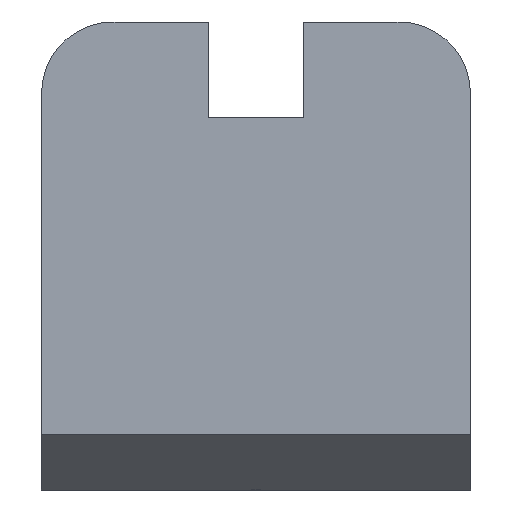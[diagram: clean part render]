
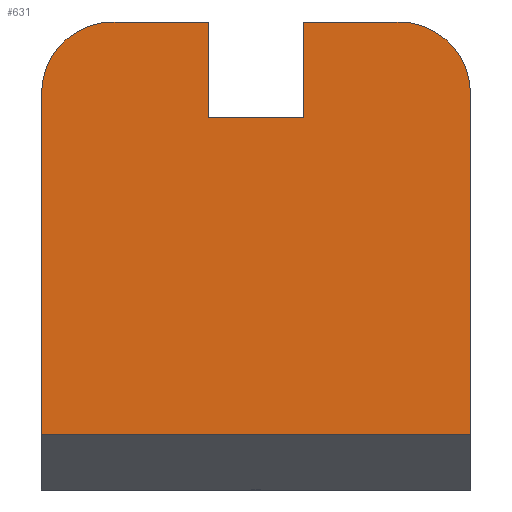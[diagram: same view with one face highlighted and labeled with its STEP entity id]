
A CAD part, top view. The second image highlights one B-rep face of the part: STEP entity #631.
In plain terms, the highlighted planar face has unit normal (0, 0, 1).
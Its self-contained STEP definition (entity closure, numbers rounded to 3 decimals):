
#15 = CARTESIAN_POINT ( 'NONE',  ( 21.823, 44.547, 4. ) ) ;
#56 = VERTEX_POINT ( 'NONE', #776 ) ;
#60 = LINE ( 'NONE', #400, #99 ) ;
#68 = EDGE_CURVE ( 'NONE', #308, #432, #564, .T. ) ;
#85 = EDGE_CURVE ( 'NONE', #425, #56, #176, .T. ) ;
#99 = VECTOR ( 'NONE', #409, 1000. ) ;
#122 = ORIENTED_EDGE ( 'NONE', *, *, #85, .T. ) ;
#123 = CIRCLE ( 'NONE', #684, 3. ) ;
#139 = ORIENTED_EDGE ( 'NONE', *, *, #194, .F. ) ;
#146 = EDGE_CURVE ( 'NONE', #341, #425, #325, .T. ) ;
#150 = VECTOR ( 'NONE', #211, 1000. ) ;
#164 = ORIENTED_EDGE ( 'NONE', *, *, #462, .T. ) ;
#174 = EDGE_CURVE ( 'NONE', #188, #56, #60, .T. ) ;
#176 = LINE ( 'NONE', #394, #235 ) ;
#185 = EDGE_CURVE ( 'NONE', #264, #188, #372, .T. ) ;
#186 = VERTEX_POINT ( 'NONE', #480 ) ;
#188 = VERTEX_POINT ( 'NONE', #617 ) ;
#194 = EDGE_CURVE ( 'NONE', #308, #264, #758, .T. ) ;
#195 = VERTEX_POINT ( 'NONE', #217 ) ;
#210 = DIRECTION ( 'NONE',  ( 1., 0., 0. ) ) ;
#211 = DIRECTION ( 'NONE',  ( 1., 0., 0. ) ) ;
#217 = CARTESIAN_POINT ( 'NONE',  ( 32.823, 31.228, 4. ) ) ;
#219 = DIRECTION ( 'NONE',  ( -1., 0., 0. ) ) ;
#225 = EDGE_CURVE ( 'NONE', #432, #186, #123, .T. ) ;
#229 = LINE ( 'NONE', #678, #709 ) ;
#235 = VECTOR ( 'NONE', #219, 1000. ) ;
#264 = VERTEX_POINT ( 'NONE', #15 ) ;
#276 = LINE ( 'NONE', #283, #579 ) ;
#280 = DIRECTION ( 'NONE',  ( 1., 0., 0. ) ) ;
#283 = CARTESIAN_POINT ( 'NONE',  ( 32.823, 31.418, 4. ) ) ;
#285 = ORIENTED_EDGE ( 'NONE', *, *, #146, .T. ) ;
#286 = CARTESIAN_POINT ( 'NONE',  ( 14.823, 48.547, 4. ) ) ;
#293 = DIRECTION ( 'NONE',  ( 0., 0., 1. ) ) ;
#296 = LINE ( 'NONE', #659, #150 ) ;
#300 = EDGE_CURVE ( 'NONE', #186, #700, #229, .T. ) ;
#305 = ORIENTED_EDGE ( 'NONE', *, *, #185, .F. ) ;
#308 = VERTEX_POINT ( 'NONE', #553 ) ;
#317 = ORIENTED_EDGE ( 'NONE', *, *, #300, .T. ) ;
#325 = CIRCLE ( 'NONE', #692, 3. ) ;
#329 = VECTOR ( 'NONE', #543, 1000. ) ;
#335 = CARTESIAN_POINT ( 'NONE',  ( 17.823, 45.547, 4. ) ) ;
#339 = CARTESIAN_POINT ( 'NONE',  ( 21.823, 44.547, 4. ) ) ;
#341 = VERTEX_POINT ( 'NONE', #348 ) ;
#348 = CARTESIAN_POINT ( 'NONE',  ( 32.823, 45.547, 4. ) ) ;
#372 = LINE ( 'NONE', #339, #477 ) ;
#394 = CARTESIAN_POINT ( 'NONE',  ( 14.823, 48.547, 4. ) ) ;
#400 = CARTESIAN_POINT ( 'NONE',  ( 25.823, 48.547, 4. ) ) ;
#405 = DIRECTION ( 'NONE',  ( 0., 0., 1. ) ) ;
#409 = DIRECTION ( 'NONE',  ( 0., 1., 0. ) ) ;
#414 = ORIENTED_EDGE ( 'NONE', *, *, #505, .T. ) ;
#419 = CARTESIAN_POINT ( 'NONE',  ( 0., 0., 4. ) ) ;
#425 = VERTEX_POINT ( 'NONE', #821 ) ;
#432 = VERTEX_POINT ( 'NONE', #472 ) ;
#450 = ORIENTED_EDGE ( 'NONE', *, *, #225, .T. ) ;
#462 = EDGE_CURVE ( 'NONE', #700, #195, #296, .T. ) ;
#472 = CARTESIAN_POINT ( 'NONE',  ( 17.823, 48.547, 4. ) ) ;
#477 = VECTOR ( 'NONE', #280, 1000. ) ;
#480 = CARTESIAN_POINT ( 'NONE',  ( 14.823, 45.547, 4. ) ) ;
#494 = FACE_OUTER_BOUND ( 'NONE', #567, .T. ) ;
#505 = EDGE_CURVE ( 'NONE', #195, #341, #276, .T. ) ;
#543 = DIRECTION ( 'NONE',  ( 0., -1., 0. ) ) ;
#545 = DIRECTION ( 'NONE',  ( -1., 0., 0. ) ) ;
#547 = AXIS2_PLACEMENT_3D ( 'NONE', #419, #293, #741 ) ;
#553 = CARTESIAN_POINT ( 'NONE',  ( 21.823, 48.547, 4. ) ) ;
#564 = LINE ( 'NONE', #286, #682 ) ;
#567 = EDGE_LOOP ( 'NONE', ( #414, #285, #122, #615, #305, #139, #632, #450, #317, #164 ) ) ;
#579 = VECTOR ( 'NONE', #669, 1000. ) ;
#615 = ORIENTED_EDGE ( 'NONE', *, *, #174, .F. ) ;
#617 = CARTESIAN_POINT ( 'NONE',  ( 25.823, 44.547, 4. ) ) ;
#631 = ADVANCED_FACE ( 'NONE', ( #494 ), #800, .T. ) ;
#632 = ORIENTED_EDGE ( 'NONE', *, *, #68, .T. ) ;
#655 = DIRECTION ( 'NONE',  ( 0., 0., 1. ) ) ;
#659 = CARTESIAN_POINT ( 'NONE',  ( 32.823, 31.228, 4. ) ) ;
#669 = DIRECTION ( 'NONE',  ( 0., 1., 0. ) ) ;
#678 = CARTESIAN_POINT ( 'NONE',  ( 14.823, 31.418, 4. ) ) ;
#680 = CARTESIAN_POINT ( 'NONE',  ( 14.823, 31.228, 4. ) ) ;
#682 = VECTOR ( 'NONE', #545, 1000. ) ;
#684 = AXIS2_PLACEMENT_3D ( 'NONE', #335, #405, #789 ) ;
#692 = AXIS2_PLACEMENT_3D ( 'NONE', #780, #655, #210 ) ;
#700 = VERTEX_POINT ( 'NONE', #680 ) ;
#709 = VECTOR ( 'NONE', #737, 1000. ) ;
#719 = CARTESIAN_POINT ( 'NONE',  ( 21.823, 48.547, 4. ) ) ;
#737 = DIRECTION ( 'NONE',  ( 0., -1., 0. ) ) ;
#741 = DIRECTION ( 'NONE',  ( 1., 0., 0. ) ) ;
#758 = LINE ( 'NONE', #719, #329 ) ;
#776 = CARTESIAN_POINT ( 'NONE',  ( 25.823, 48.547, 4. ) ) ;
#780 = CARTESIAN_POINT ( 'NONE',  ( 29.823, 45.547, 4. ) ) ;
#789 = DIRECTION ( 'NONE',  ( 1., 0., 0. ) ) ;
#800 = PLANE ( 'NONE',  #547 ) ;
#821 = CARTESIAN_POINT ( 'NONE',  ( 29.823, 48.547, 4. ) ) ;
